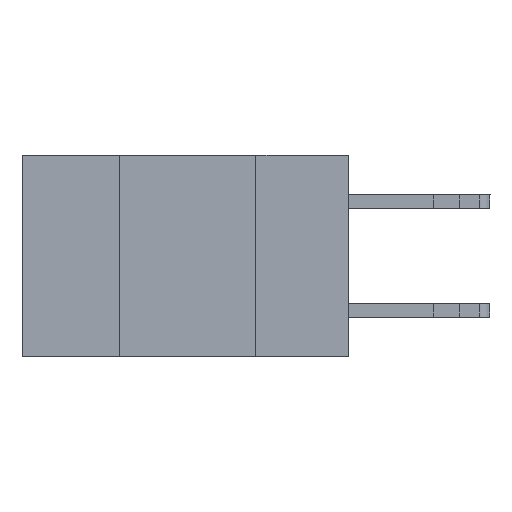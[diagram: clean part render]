
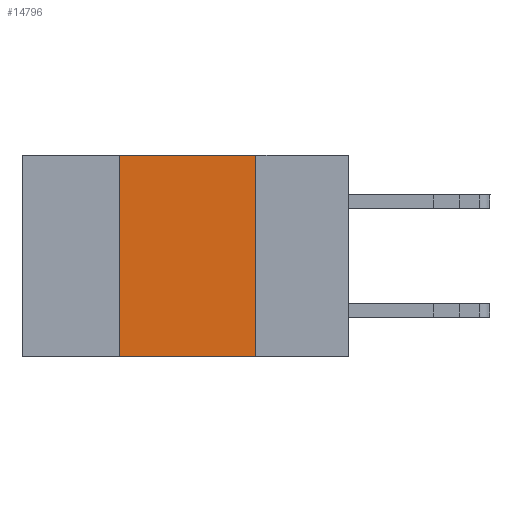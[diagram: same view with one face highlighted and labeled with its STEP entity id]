
A CAD part, left-side view. The second image highlights one B-rep face of the part: STEP entity #14796.
In plain terms, the highlighted planar face has unit normal (-1, 0, 0).
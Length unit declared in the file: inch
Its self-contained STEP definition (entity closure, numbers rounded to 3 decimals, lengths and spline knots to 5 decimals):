
#639 = ORIENTED_EDGE ( 'NONE', *, *, #14550, .F. ) ;
#818 = CARTESIAN_POINT ( 'NONE',  ( 0., 0.6, -0.37 ) ) ;
#2537 = AXIS2_PLACEMENT_3D ( 'NONE', #9944, #17206, #10047 ) ;
#2545 = CARTESIAN_POINT ( 'NONE',  ( 0., 0.42, -0.37 ) ) ;
#3139 = DIRECTION ( 'NONE',  ( 0., 0., -1. ) ) ;
#4046 = LINE ( 'NONE', #8509, #12168 ) ;
#4064 = VECTOR ( 'NONE', #3139, 39.37008 ) ;
#5062 = EDGE_CURVE ( 'NONE', #18301, #12660, #9619, .T. ) ;
#8509 = CARTESIAN_POINT ( 'NONE',  ( 0., 0.42, 0. ) ) ;
#8512 = LINE ( 'NONE', #17770, #9805 ) ;
#8906 = EDGE_LOOP ( 'NONE', ( #16651, #13810, #639, #12389 ) ) ;
#9238 = VERTEX_POINT ( 'NONE', #18509 ) ;
#9619 = LINE ( 'NONE', #818, #15829 ) ;
#9805 = VECTOR ( 'NONE', #15709, 39.37008 ) ;
#9944 = CARTESIAN_POINT ( 'NONE',  ( 0., 0.6, 0. ) ) ;
#10047 = DIRECTION ( 'NONE',  ( 0., 0., -1. ) ) ;
#11025 = EDGE_CURVE ( 'NONE', #12696, #9238, #8512, .T. ) ;
#11392 = DIRECTION ( 'NONE',  ( 0., -1., 0. ) ) ;
#12168 = VECTOR ( 'NONE', #17430, 39.37008 ) ;
#12389 = ORIENTED_EDGE ( 'NONE', *, *, #5062, .T. ) ;
#12660 = VERTEX_POINT ( 'NONE', #15680 ) ;
#12696 = VERTEX_POINT ( 'NONE', #12794 ) ;
#12794 = CARTESIAN_POINT ( 'NONE',  ( 0., 0.42, 0. ) ) ;
#13810 = ORIENTED_EDGE ( 'NONE', *, *, #11025, .F. ) ;
#14550 = EDGE_CURVE ( 'NONE', #18301, #12696, #4046, .T. ) ;
#14796 = ADVANCED_FACE ( 'NONE', ( #15979 ), #17003, .F. ) ;
#15680 = CARTESIAN_POINT ( 'NONE',  ( 0., 0.17, -0.37 ) ) ;
#15709 = DIRECTION ( 'NONE',  ( 0., -1., 0. ) ) ;
#15829 = VECTOR ( 'NONE', #11392, 39.37008 ) ;
#15979 = FACE_OUTER_BOUND ( 'NONE', #8906, .T. ) ;
#16131 = EDGE_CURVE ( 'NONE', #9238, #12660, #17768, .T. ) ;
#16422 = CARTESIAN_POINT ( 'NONE',  ( 0., 0.17, 0. ) ) ;
#16651 = ORIENTED_EDGE ( 'NONE', *, *, #16131, .F. ) ;
#17003 = PLANE ( 'NONE',  #2537 ) ;
#17206 = DIRECTION ( 'NONE',  ( 1., 0., 0. ) ) ;
#17430 = DIRECTION ( 'NONE',  ( 0., 0., 1. ) ) ;
#17768 = LINE ( 'NONE', #16422, #4064 ) ;
#17770 = CARTESIAN_POINT ( 'NONE',  ( 0., 0.6, 0. ) ) ;
#18301 = VERTEX_POINT ( 'NONE', #2545 ) ;
#18509 = CARTESIAN_POINT ( 'NONE',  ( 0., 0.17, 0. ) ) ;
